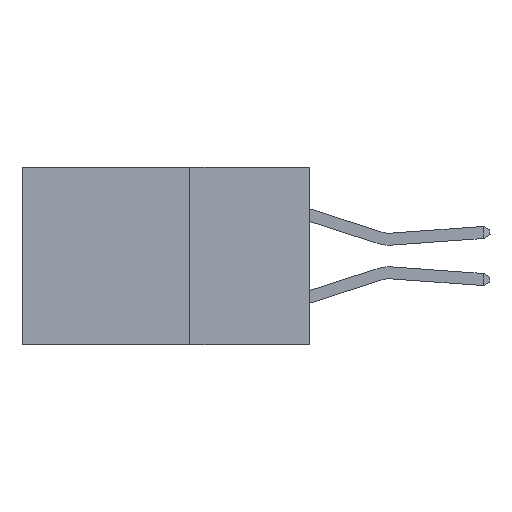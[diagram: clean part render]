
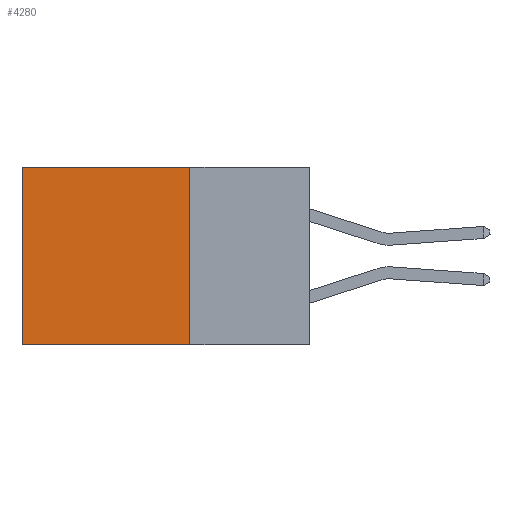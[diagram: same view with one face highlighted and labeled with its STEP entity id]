
A CAD part, left-side view. The second image highlights one B-rep face of the part: STEP entity #4280.
In plain terms, the highlighted planar face has unit normal (-1, 0, 0).
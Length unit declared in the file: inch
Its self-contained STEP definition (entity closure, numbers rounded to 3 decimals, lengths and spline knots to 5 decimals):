
#15 = VECTOR ( 'NONE', #2507, 39.37008 ) ;
#1223 = DIRECTION ( 'NONE',  ( 0., 1., 0. ) ) ;
#1349 = DIRECTION ( 'NONE',  ( 0., 0., -1. ) ) ;
#2240 = EDGE_CURVE ( 'NONE', #7461, #13772, #9296, .T. ) ;
#2358 = CARTESIAN_POINT ( 'NONE',  ( 0.2615, 0.25, -0.37 ) ) ;
#2507 = DIRECTION ( 'NONE',  ( 0., 0., -1. ) ) ;
#3129 = VECTOR ( 'NONE', #1349, 39.37008 ) ;
#3193 = CARTESIAN_POINT ( 'NONE',  ( 0.2615, 0.25, -0.37 ) ) ;
#3389 = LINE ( 'NONE', #4522, #3129 ) ;
#3661 = ORIENTED_EDGE ( 'NONE', *, *, #13458, .F. ) ;
#4280 = ADVANCED_FACE ( 'NONE', ( #10766 ), #11747, .F. ) ;
#4522 = CARTESIAN_POINT ( 'NONE',  ( 0.2615, 0.6, -0.37 ) ) ;
#4603 = CARTESIAN_POINT ( 'NONE',  ( 0.2615, 0.25, 0. ) ) ;
#4690 = LINE ( 'NONE', #2358, #15 ) ;
#5394 = ORIENTED_EDGE ( 'NONE', *, *, #10086, .T. ) ;
#6155 = ORIENTED_EDGE ( 'NONE', *, *, #2240, .F. ) ;
#6254 = VECTOR ( 'NONE', #1223, 39.37008 ) ;
#6337 = EDGE_LOOP ( 'NONE', ( #7526, #6155, #3661, #5394 ) ) ;
#6442 = DIRECTION ( 'NONE',  ( 0., 0., -1. ) ) ;
#7266 = VECTOR ( 'NONE', #7390, 39.37008 ) ;
#7390 = DIRECTION ( 'NONE',  ( 0., 1., 0. ) ) ;
#7461 = VERTEX_POINT ( 'NONE', #7772 ) ;
#7526 = ORIENTED_EDGE ( 'NONE', *, *, #11701, .T. ) ;
#7731 = LINE ( 'NONE', #4603, #6254 ) ;
#7772 = CARTESIAN_POINT ( 'NONE',  ( 0.2615, 0.25, -0.37 ) ) ;
#8367 = CARTESIAN_POINT ( 'NONE',  ( 0.2615, 0.25, 0. ) ) ;
#8526 = CARTESIAN_POINT ( 'NONE',  ( 0.2615, 0.25, -0.37 ) ) ;
#9296 = LINE ( 'NONE', #8526, #7266 ) ;
#9406 = CARTESIAN_POINT ( 'NONE',  ( 0.2615, 0.6, 0. ) ) ;
#10086 = EDGE_CURVE ( 'NONE', #11214, #10336, #7731, .T. ) ;
#10336 = VERTEX_POINT ( 'NONE', #9406 ) ;
#10766 = FACE_OUTER_BOUND ( 'NONE', #6337, .T. ) ;
#11214 = VERTEX_POINT ( 'NONE', #8367 ) ;
#11701 = EDGE_CURVE ( 'NONE', #10336, #13772, #3389, .T. ) ;
#11747 = PLANE ( 'NONE',  #12035 ) ;
#11812 = DIRECTION ( 'NONE',  ( 1., 0., 0. ) ) ;
#12035 = AXIS2_PLACEMENT_3D ( 'NONE', #3193, #11812, #6442 ) ;
#12645 = CARTESIAN_POINT ( 'NONE',  ( 0.2615, 0.6, -0.37 ) ) ;
#13458 = EDGE_CURVE ( 'NONE', #11214, #7461, #4690, .T. ) ;
#13772 = VERTEX_POINT ( 'NONE', #12645 ) ;
